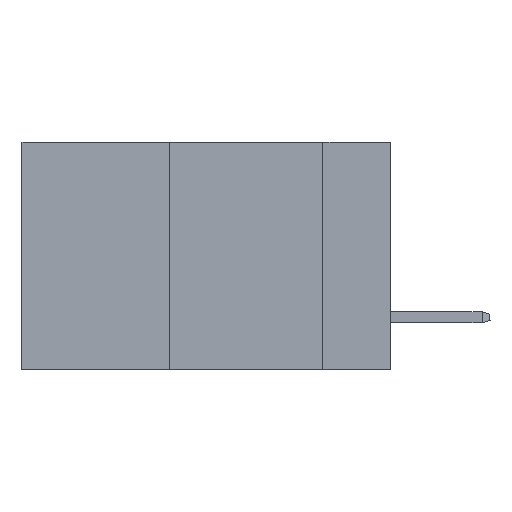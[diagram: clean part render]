
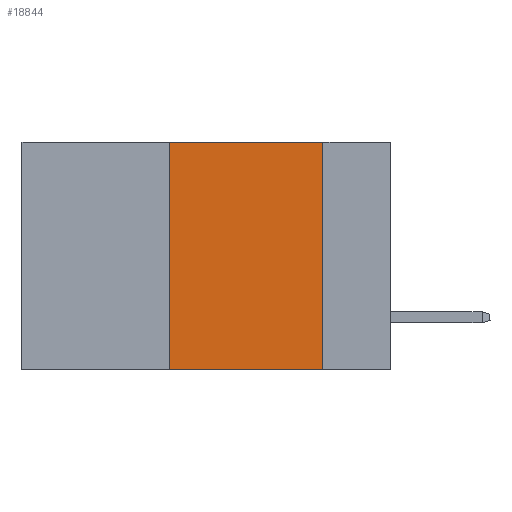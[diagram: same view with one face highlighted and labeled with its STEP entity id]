
A CAD part, left-side view. The second image highlights one B-rep face of the part: STEP entity #18844.
In plain terms, the highlighted planar face has unit normal (-1, 0, 0).
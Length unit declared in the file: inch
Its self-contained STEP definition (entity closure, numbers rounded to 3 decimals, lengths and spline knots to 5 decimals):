
#219 = DIRECTION ( 'NONE',  ( 1., 0., 0. ) ) ;
#412 = VERTEX_POINT ( 'NONE', #10869 ) ;
#442 = CARTESIAN_POINT ( 'NONE',  ( 0., 0.36, -0.37 ) ) ;
#1926 = PLANE ( 'NONE',  #17277 ) ;
#2453 = DIRECTION ( 'NONE',  ( 0., -1., 0. ) ) ;
#3643 = DIRECTION ( 'NONE',  ( 0., 0., -1. ) ) ;
#4432 = ORIENTED_EDGE ( 'NONE', *, *, #4760, .T. ) ;
#4760 = EDGE_CURVE ( 'NONE', #10201, #4909, #10790, .T. ) ;
#4909 = VERTEX_POINT ( 'NONE', #6934 ) ;
#4939 = DIRECTION ( 'NONE',  ( 0., 0., -1. ) ) ;
#5209 = VECTOR ( 'NONE', #15452, 39.37008 ) ;
#6222 = FACE_OUTER_BOUND ( 'NONE', #12012, .T. ) ;
#6516 = CARTESIAN_POINT ( 'NONE',  ( 0., 0.11, 0. ) ) ;
#6610 = LINE ( 'NONE', #6516, #16176 ) ;
#6772 = VECTOR ( 'NONE', #8323, 39.37008 ) ;
#6934 = CARTESIAN_POINT ( 'NONE',  ( 0., 0.11, -0.37 ) ) ;
#7718 = EDGE_CURVE ( 'NONE', #412, #16168, #15015, .T. ) ;
#8323 = DIRECTION ( 'NONE',  ( 0., -1., 0. ) ) ;
#8666 = ORIENTED_EDGE ( 'NONE', *, *, #7718, .F. ) ;
#9107 = EDGE_CURVE ( 'NONE', #10201, #412, #12704, .T. ) ;
#10036 = ORIENTED_EDGE ( 'NONE', *, *, #16149, .F. ) ;
#10201 = VERTEX_POINT ( 'NONE', #442 ) ;
#10790 = LINE ( 'NONE', #20713, #17547 ) ;
#10869 = CARTESIAN_POINT ( 'NONE',  ( 0., 0.36, 0. ) ) ;
#12012 = EDGE_LOOP ( 'NONE', ( #10036, #8666, #16069, #4432 ) ) ;
#12704 = LINE ( 'NONE', #17315, #5209 ) ;
#13118 = CARTESIAN_POINT ( 'NONE',  ( 0., 0.6, 0. ) ) ;
#15015 = LINE ( 'NONE', #13118, #6772 ) ;
#15452 = DIRECTION ( 'NONE',  ( 0., 0., 1. ) ) ;
#16069 = ORIENTED_EDGE ( 'NONE', *, *, #9107, .F. ) ;
#16149 = EDGE_CURVE ( 'NONE', #16168, #4909, #6610, .T. ) ;
#16168 = VERTEX_POINT ( 'NONE', #19804 ) ;
#16176 = VECTOR ( 'NONE', #4939, 39.37008 ) ;
#16799 = CARTESIAN_POINT ( 'NONE',  ( 0., 0.6, 0. ) ) ;
#17277 = AXIS2_PLACEMENT_3D ( 'NONE', #16799, #219, #3643 ) ;
#17315 = CARTESIAN_POINT ( 'NONE',  ( 0., 0.36, 0. ) ) ;
#17547 = VECTOR ( 'NONE', #2453, 39.37008 ) ;
#18844 = ADVANCED_FACE ( 'NONE', ( #6222 ), #1926, .F. ) ;
#19804 = CARTESIAN_POINT ( 'NONE',  ( 0., 0.11, 0. ) ) ;
#20713 = CARTESIAN_POINT ( 'NONE',  ( 0., 0.6, -0.37 ) ) ;
